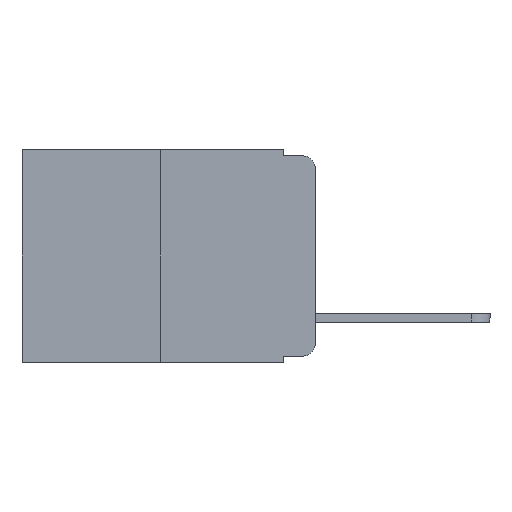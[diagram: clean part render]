
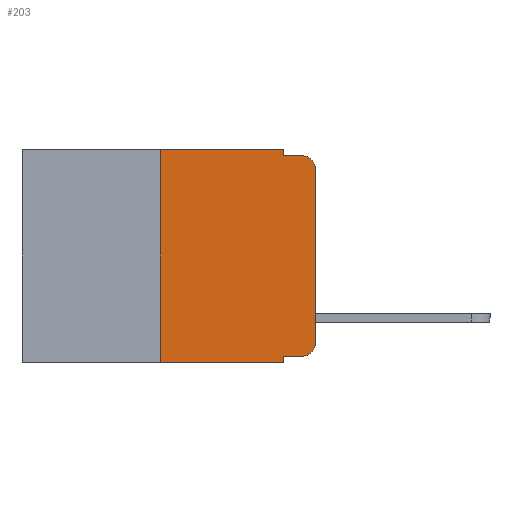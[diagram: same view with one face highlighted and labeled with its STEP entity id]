
A CAD part, left-side view. The second image highlights one B-rep face of the part: STEP entity #203.
In plain terms, the highlighted planar face has unit normal (-1, 0, 0).
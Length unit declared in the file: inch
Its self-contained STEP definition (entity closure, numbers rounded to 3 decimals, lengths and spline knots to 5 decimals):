
#70 = LINE ( 'NONE', #4933, #1888 ) ;
#117 = CARTESIAN_POINT ( 'NONE',  ( 0., 0.473, 0. ) ) ;
#203 = ADVANCED_FACE ( 'NONE', ( #4152 ), #1144, .F. ) ;
#309 = EDGE_CURVE ( 'NONE', #2775, #6394, #7193, .T. ) ;
#375 = DIRECTION ( 'NONE',  ( 0., 0., -1. ) ) ;
#384 = DIRECTION ( 'NONE',  ( 1., 0., 0. ) ) ;
#457 = VERTEX_POINT ( 'NONE', #8016 ) ;
#461 = CIRCLE ( 'NONE', #6239, 0.02 ) ;
#570 = CARTESIAN_POINT ( 'NONE',  ( 0., 0., 0. ) ) ;
#742 = CARTESIAN_POINT ( 'NONE',  ( 0., 0.02, -0.313 ) ) ;
#899 = CARTESIAN_POINT ( 'NONE',  ( 0., 0.051, -0.333 ) ) ;
#944 = CARTESIAN_POINT ( 'NONE',  ( 0., 0.473, 0. ) ) ;
#962 = CARTESIAN_POINT ( 'NONE',  ( 0., 0.051, -0.343 ) ) ;
#1070 = VERTEX_POINT ( 'NONE', #1167 ) ;
#1075 = LINE ( 'NONE', #570, #6663 ) ;
#1111 = EDGE_CURVE ( 'NONE', #2775, #3896, #1831, .T. ) ;
#1117 = VECTOR ( 'NONE', #2268, 39.37008 ) ;
#1144 = PLANE ( 'NONE',  #6577 ) ;
#1165 = VERTEX_POINT ( 'NONE', #899 ) ;
#1167 = CARTESIAN_POINT ( 'NONE',  ( 0., 0.02, -0.333 ) ) ;
#1170 = ORIENTED_EDGE ( 'NONE', *, *, #5216, .T. ) ;
#1248 = AXIS2_PLACEMENT_3D ( 'NONE', #4626, #2443, #5457 ) ;
#1272 = LINE ( 'NONE', #944, #9105 ) ;
#1831 = LINE ( 'NONE', #2881, #3877 ) ;
#1888 = VECTOR ( 'NONE', #9394, 39.37008 ) ;
#1966 = DIRECTION ( 'NONE',  ( 0., 0., 1. ) ) ;
#1991 = ORIENTED_EDGE ( 'NONE', *, *, #8726, .F. ) ;
#2268 = DIRECTION ( 'NONE',  ( 0., -1., 0. ) ) ;
#2443 = DIRECTION ( 'NONE',  ( -1., 0., 0. ) ) ;
#2510 = VERTEX_POINT ( 'NONE', #7605 ) ;
#2735 = EDGE_CURVE ( 'NONE', #5854, #3720, #1075, .T. ) ;
#2754 = EDGE_LOOP ( 'NONE', ( #7602, #4383, #8739, #7218, #6656, #6435, #3038, #1991, #1170, #4064 ) ) ;
#2775 = VERTEX_POINT ( 'NONE', #3694 ) ;
#2881 = CARTESIAN_POINT ( 'NONE',  ( 0., 0.25, 0. ) ) ;
#3007 = EDGE_CURVE ( 'NONE', #1070, #5854, #461, .T. ) ;
#3038 = ORIENTED_EDGE ( 'NONE', *, *, #309, .T. ) ;
#3204 = VECTOR ( 'NONE', #8173, 39.37008 ) ;
#3378 = EDGE_CURVE ( 'NONE', #3720, #8538, #5010, .T. ) ;
#3694 = CARTESIAN_POINT ( 'NONE',  ( 0., 0.25, -0.343 ) ) ;
#3695 = CARTESIAN_POINT ( 'NONE',  ( 0., 0.25, 0. ) ) ;
#3720 = VERTEX_POINT ( 'NONE', #4510 ) ;
#3877 = VECTOR ( 'NONE', #8578, 39.37008 ) ;
#3896 = VERTEX_POINT ( 'NONE', #3695 ) ;
#3988 = CARTESIAN_POINT ( 'NONE',  ( 0., 0.02, -0.01 ) ) ;
#4064 = ORIENTED_EDGE ( 'NONE', *, *, #3007, .T. ) ;
#4152 = FACE_OUTER_BOUND ( 'NONE', #2754, .T. ) ;
#4383 = ORIENTED_EDGE ( 'NONE', *, *, #3378, .T. ) ;
#4510 = CARTESIAN_POINT ( 'NONE',  ( 0., 0., -0.03 ) ) ;
#4626 = CARTESIAN_POINT ( 'NONE',  ( 0., 0.02, -0.03 ) ) ;
#4933 = CARTESIAN_POINT ( 'NONE',  ( 0., 0.051, 0. ) ) ;
#5010 = CIRCLE ( 'NONE', #1248, 0.02 ) ;
#5216 = EDGE_CURVE ( 'NONE', #1165, #1070, #9390, .T. ) ;
#5457 = DIRECTION ( 'NONE',  ( 0., 0., -1. ) ) ;
#5651 = DIRECTION ( 'NONE',  ( 0., 0., -1. ) ) ;
#5854 = VERTEX_POINT ( 'NONE', #9329 ) ;
#6239 = AXIS2_PLACEMENT_3D ( 'NONE', #742, #8652, #7741 ) ;
#6394 = VERTEX_POINT ( 'NONE', #962 ) ;
#6435 = ORIENTED_EDGE ( 'NONE', *, *, #1111, .F. ) ;
#6515 = DIRECTION ( 'NONE',  ( 0., -1., 0. ) ) ;
#6534 = VECTOR ( 'NONE', #5651, 39.37008 ) ;
#6577 = AXIS2_PLACEMENT_3D ( 'NONE', #117, #384, #375 ) ;
#6656 = ORIENTED_EDGE ( 'NONE', *, *, #8590, .F. ) ;
#6663 = VECTOR ( 'NONE', #1966, 39.37008 ) ;
#6896 = VECTOR ( 'NONE', #6515, 39.37008 ) ;
#7193 = LINE ( 'NONE', #7364, #3204 ) ;
#7218 = ORIENTED_EDGE ( 'NONE', *, *, #7601, .F. ) ;
#7364 = CARTESIAN_POINT ( 'NONE',  ( 0., 0.473, -0.343 ) ) ;
#7601 = EDGE_CURVE ( 'NONE', #457, #2510, #8540, .T. ) ;
#7602 = ORIENTED_EDGE ( 'NONE', *, *, #2735, .T. ) ;
#7605 = CARTESIAN_POINT ( 'NONE',  ( 0., 0.051, -0.01 ) ) ;
#7655 = CARTESIAN_POINT ( 'NONE',  ( 0., 0.051, -0.333 ) ) ;
#7741 = DIRECTION ( 'NONE',  ( 0., 0., -1. ) ) ;
#7742 = EDGE_CURVE ( 'NONE', #2510, #8538, #9127, .T. ) ;
#8016 = CARTESIAN_POINT ( 'NONE',  ( 0., 0.051, 0. ) ) ;
#8173 = DIRECTION ( 'NONE',  ( 0., -1., 0. ) ) ;
#8537 = DIRECTION ( 'NONE',  ( 0., -1., 0. ) ) ;
#8538 = VERTEX_POINT ( 'NONE', #3988 ) ;
#8540 = LINE ( 'NONE', #8623, #6534 ) ;
#8578 = DIRECTION ( 'NONE',  ( 0., 0., 1. ) ) ;
#8590 = EDGE_CURVE ( 'NONE', #3896, #457, #1272, .T. ) ;
#8623 = CARTESIAN_POINT ( 'NONE',  ( 0., 0.051, 0. ) ) ;
#8652 = DIRECTION ( 'NONE',  ( -1., 0., 0. ) ) ;
#8726 = EDGE_CURVE ( 'NONE', #1165, #6394, #70, .T. ) ;
#8739 = ORIENTED_EDGE ( 'NONE', *, *, #7742, .F. ) ;
#9105 = VECTOR ( 'NONE', #8537, 39.37008 ) ;
#9127 = LINE ( 'NONE', #9514, #6896 ) ;
#9329 = CARTESIAN_POINT ( 'NONE',  ( 0., 0., -0.313 ) ) ;
#9390 = LINE ( 'NONE', #7655, #1117 ) ;
#9394 = DIRECTION ( 'NONE',  ( 0., 0., -1. ) ) ;
#9514 = CARTESIAN_POINT ( 'NONE',  ( 0., 0.051, -0.01 ) ) ;
